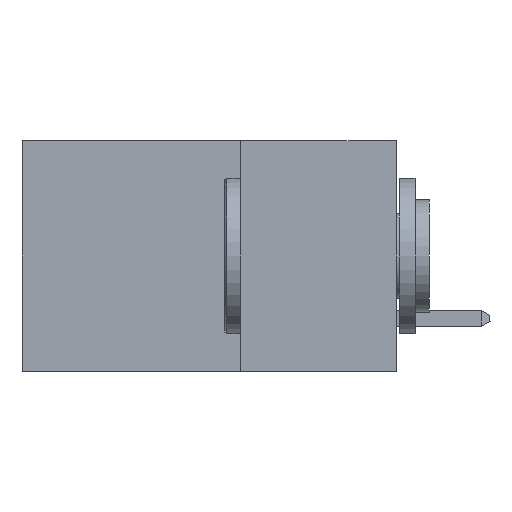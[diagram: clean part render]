
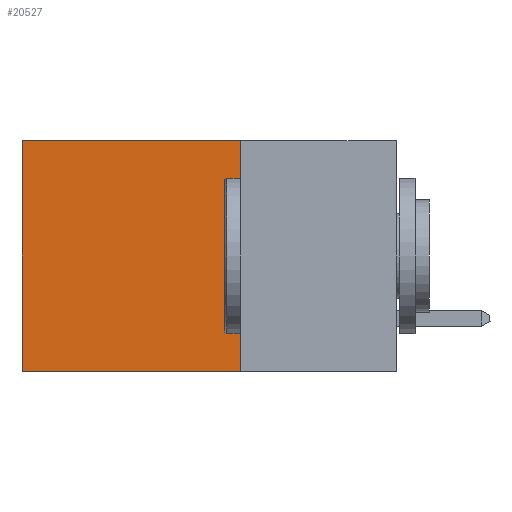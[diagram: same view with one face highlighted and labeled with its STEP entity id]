
A CAD part, left-side view. The second image highlights one B-rep face of the part: STEP entity #20527.
In plain terms, the highlighted planar face has unit normal (-1, 0, 0).
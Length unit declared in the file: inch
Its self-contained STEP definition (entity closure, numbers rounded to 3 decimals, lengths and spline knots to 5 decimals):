
#327 = LINE ( 'NONE', #21049, #8063 ) ;
#2329 = EDGE_CURVE ( 'NONE', #13683, #3016, #327, .T. ) ;
#2542 = FACE_OUTER_BOUND ( 'NONE', #14421, .T. ) ;
#3016 = VERTEX_POINT ( 'NONE', #11285 ) ;
#4213 = PLANE ( 'NONE',  #10170 ) ;
#5420 = DIRECTION ( 'NONE',  ( 0., 0., -1. ) ) ;
#5562 = CARTESIAN_POINT ( 'NONE',  ( 0.298, 0.6, 0. ) ) ;
#5747 = VECTOR ( 'NONE', #5420, 39.37008 ) ;
#5936 = CARTESIAN_POINT ( 'NONE',  ( 0.298, 0.25, -0.37 ) ) ;
#7256 = CARTESIAN_POINT ( 'NONE',  ( 0.298, 0.25, 0. ) ) ;
#7563 = DIRECTION ( 'NONE',  ( 0., 1., 0. ) ) ;
#8063 = VECTOR ( 'NONE', #20445, 39.37008 ) ;
#8105 = CARTESIAN_POINT ( 'NONE',  ( 0.298, 0.6, 0. ) ) ;
#9167 = ORIENTED_EDGE ( 'NONE', *, *, #22076, .T. ) ;
#10170 = AXIS2_PLACEMENT_3D ( 'NONE', #17693, #14177, #10843 ) ;
#10205 = EDGE_CURVE ( 'NONE', #3016, #20375, #21374, .T. ) ;
#10843 = DIRECTION ( 'NONE',  ( 0., 0., -1. ) ) ;
#11055 = EDGE_CURVE ( 'NONE', #13683, #19106, #11744, .T. ) ;
#11285 = CARTESIAN_POINT ( 'NONE',  ( 0.298, 0.25, -0.37 ) ) ;
#11744 = LINE ( 'NONE', #7256, #19202 ) ;
#12421 = ORIENTED_EDGE ( 'NONE', *, *, #10205, .F. ) ;
#13187 = LINE ( 'NONE', #5562, #5747 ) ;
#13683 = VERTEX_POINT ( 'NONE', #15398 ) ;
#14106 = CARTESIAN_POINT ( 'NONE',  ( 0.298, 0.6, -0.37 ) ) ;
#14177 = DIRECTION ( 'NONE',  ( 1., 0., 0. ) ) ;
#14421 = EDGE_LOOP ( 'NONE', ( #9167, #12421, #15568, #21568 ) ) ;
#15398 = CARTESIAN_POINT ( 'NONE',  ( 0.298, 0.25, 0. ) ) ;
#15546 = VECTOR ( 'NONE', #7563, 39.37008 ) ;
#15568 = ORIENTED_EDGE ( 'NONE', *, *, #2329, .F. ) ;
#17384 = DIRECTION ( 'NONE',  ( 0., 1., 0. ) ) ;
#17693 = CARTESIAN_POINT ( 'NONE',  ( 0.298, 0.25, 0. ) ) ;
#19106 = VERTEX_POINT ( 'NONE', #8105 ) ;
#19202 = VECTOR ( 'NONE', #17384, 39.37008 ) ;
#20375 = VERTEX_POINT ( 'NONE', #14106 ) ;
#20445 = DIRECTION ( 'NONE',  ( 0., 0., -1. ) ) ;
#20527 = ADVANCED_FACE ( 'NONE', ( #2542 ), #4213, .F. ) ;
#21049 = CARTESIAN_POINT ( 'NONE',  ( 0.298, 0.25, 0. ) ) ;
#21374 = LINE ( 'NONE', #5936, #15546 ) ;
#21568 = ORIENTED_EDGE ( 'NONE', *, *, #11055, .T. ) ;
#22076 = EDGE_CURVE ( 'NONE', #19106, #20375, #13187, .T. ) ;
